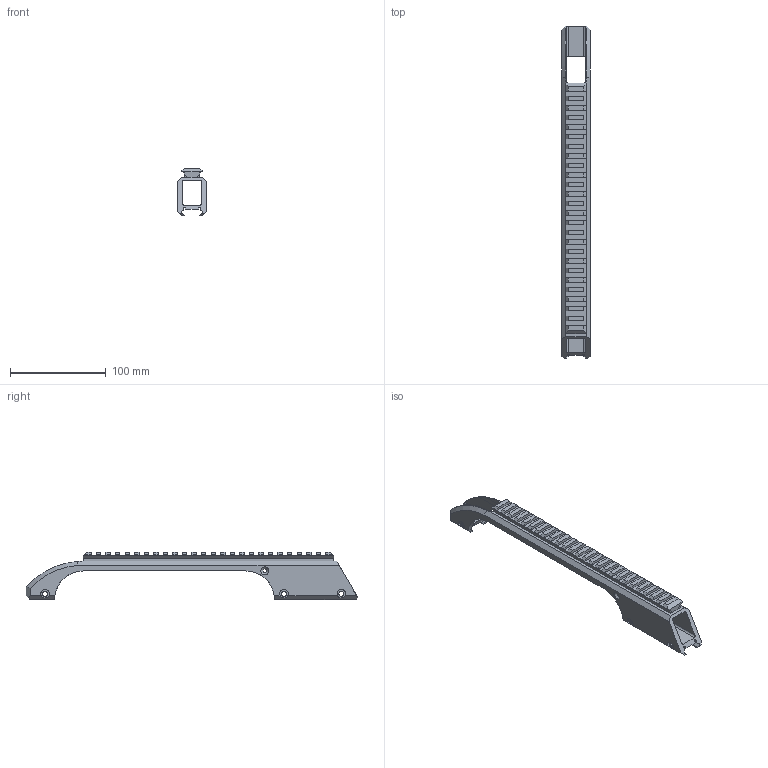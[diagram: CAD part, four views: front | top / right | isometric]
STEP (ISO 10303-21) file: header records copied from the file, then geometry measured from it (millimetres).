
FILE_DESCRIPTION(('FreeCAD Model'),'2;1');
FILE_NAME('Open CASCADE Shape Model','2025-08-02T21:24:23',(''),(''), 'Open CASCADE STEP processor 7.8','FreeCAD','Unknown');
FILE_SCHEMA(('AUTOMOTIVE_DESIGN { 1 0 10303 214 1 1 1 1 }'));
Length unit declared in the file: millimetre
Products named in the file (1): difference004
Bounding box: 30 x 347.47 x 49.4 mm (x, y, z)
Volume: 116563.1 mm3; surface area: 54584.2 mm2
Topology: 1 solids, 1 shells, 320 faces, 959 edges, 632 vertices
Faces by surface type: plane 284, cylinder 32, cone 4
Full cylindrical faces by diameter (mm): 4.4 x2, 5.2 x6, 8.4 x2
Entity records: 11305 total; most frequent: CARTESIAN_POINT 2536, ORIENTED_EDGE 1918, DIRECTION 1717, EDGE_CURVE 959, LINE 795, VECTOR 795, VERTEX_POINT 632, AXIS2_PLACEMENT_3D 461
